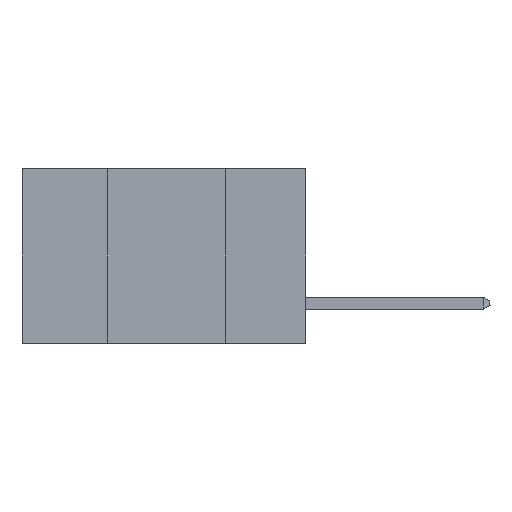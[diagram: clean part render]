
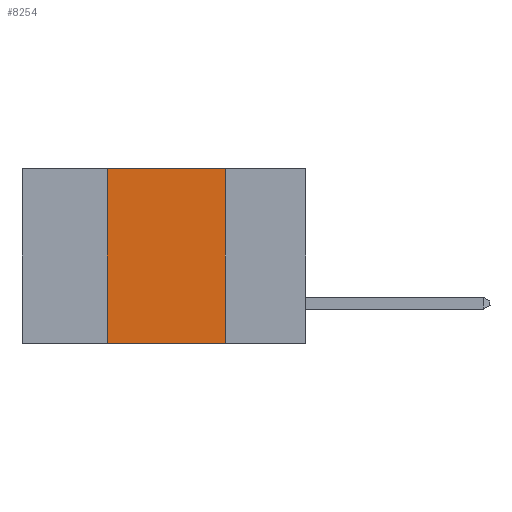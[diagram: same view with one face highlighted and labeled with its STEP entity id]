
A CAD part, left-side view. The second image highlights one B-rep face of the part: STEP entity #8254.
In plain terms, the highlighted planar face has unit normal (-1, 0, 0).
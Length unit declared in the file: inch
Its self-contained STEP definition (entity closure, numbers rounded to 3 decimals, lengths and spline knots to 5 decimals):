
#787 = VERTEX_POINT ( 'NONE', #10997 ) ;
#1899 = ORIENTED_EDGE ( 'NONE', *, *, #10352, .F. ) ;
#2003 = DIRECTION ( 'NONE',  ( 0., -1., 0. ) ) ;
#2013 = VECTOR ( 'NONE', #12650, 39.37008 ) ;
#2204 = DIRECTION ( 'NONE',  ( 0., 0., 1. ) ) ;
#2331 = AXIS2_PLACEMENT_3D ( 'NONE', #12468, #15111, #12832 ) ;
#2682 = ORIENTED_EDGE ( 'NONE', *, *, #12955, .F. ) ;
#4128 = PLANE ( 'NONE',  #2331 ) ;
#4597 = CARTESIAN_POINT ( 'NONE',  ( 0., 0.42, 0. ) ) ;
#4747 = VECTOR ( 'NONE', #8186, 39.37008 ) ;
#4813 = ORIENTED_EDGE ( 'NONE', *, *, #13580, .T. ) ;
#5830 = EDGE_LOOP ( 'NONE', ( #1899, #9241, #2682, #4813 ) ) ;
#5895 = LINE ( 'NONE', #13762, #11077 ) ;
#5908 = CARTESIAN_POINT ( 'NONE',  ( 0., 0.42, -0.37 ) ) ;
#7053 = CARTESIAN_POINT ( 'NONE',  ( 0., 0.42, 0. ) ) ;
#8186 = DIRECTION ( 'NONE',  ( 0., -1., 0. ) ) ;
#8254 = ADVANCED_FACE ( 'NONE', ( #11569 ), #4128, .F. ) ;
#8721 = LINE ( 'NONE', #10552, #2013 ) ;
#9241 = ORIENTED_EDGE ( 'NONE', *, *, #12820, .F. ) ;
#9314 = VERTEX_POINT ( 'NONE', #5908 ) ;
#10352 = EDGE_CURVE ( 'NONE', #787, #12748, #8721, .T. ) ;
#10517 = LINE ( 'NONE', #14207, #4747 ) ;
#10521 = VERTEX_POINT ( 'NONE', #7053 ) ;
#10552 = CARTESIAN_POINT ( 'NONE',  ( 0., 0.17, 0. ) ) ;
#10894 = VECTOR ( 'NONE', #2204, 39.37008 ) ;
#10997 = CARTESIAN_POINT ( 'NONE',  ( 0., 0.17, 0. ) ) ;
#11077 = VECTOR ( 'NONE', #2003, 39.37008 ) ;
#11569 = FACE_OUTER_BOUND ( 'NONE', #5830, .T. ) ;
#12468 = CARTESIAN_POINT ( 'NONE',  ( 0., 0.6, 0. ) ) ;
#12650 = DIRECTION ( 'NONE',  ( 0., 0., -1. ) ) ;
#12681 = CARTESIAN_POINT ( 'NONE',  ( 0., 0.17, -0.37 ) ) ;
#12748 = VERTEX_POINT ( 'NONE', #12681 ) ;
#12820 = EDGE_CURVE ( 'NONE', #10521, #787, #5895, .T. ) ;
#12832 = DIRECTION ( 'NONE',  ( 0., 0., -1. ) ) ;
#12955 = EDGE_CURVE ( 'NONE', #9314, #10521, #13849, .T. ) ;
#13580 = EDGE_CURVE ( 'NONE', #9314, #12748, #10517, .T. ) ;
#13762 = CARTESIAN_POINT ( 'NONE',  ( 0., 0.6, 0. ) ) ;
#13849 = LINE ( 'NONE', #4597, #10894 ) ;
#14207 = CARTESIAN_POINT ( 'NONE',  ( 0., 0.6, -0.37 ) ) ;
#15111 = DIRECTION ( 'NONE',  ( 1., 0., 0. ) ) ;
